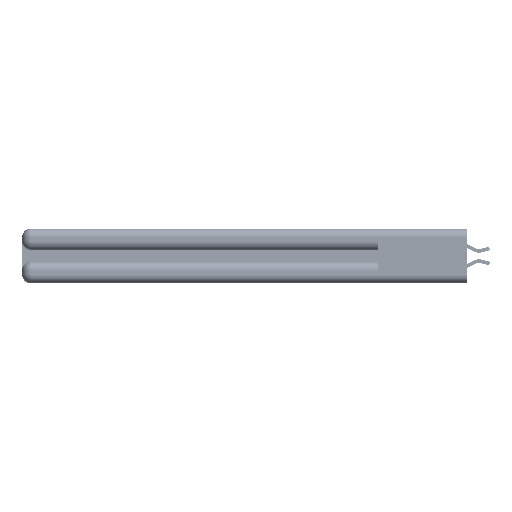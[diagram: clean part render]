
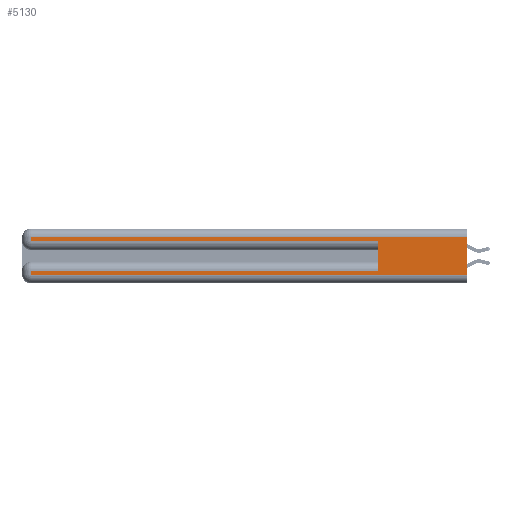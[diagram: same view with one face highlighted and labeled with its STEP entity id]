
A CAD part, left-side view. The second image highlights one B-rep face of the part: STEP entity #5130.
In plain terms, the highlighted planar face has unit normal (-1, 0, 0).
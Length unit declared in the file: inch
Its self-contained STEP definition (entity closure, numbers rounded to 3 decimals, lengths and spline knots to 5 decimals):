
#1641 = VECTOR ( 'NONE', #52643, 39.37008 ) ;
#1784 = VERTEX_POINT ( 'NONE', #21558 ) ;
#3058 = EDGE_CURVE ( 'NONE', #45789, #15807, #40304, .T. ) ;
#3540 = VERTEX_POINT ( 'NONE', #5433 ) ;
#3769 = DIRECTION ( 'NONE',  ( 0., 0., 1. ) ) ;
#5130 = ADVANCED_FACE ( 'NONE', ( #40050 ), #31026, .F. ) ;
#5433 = CARTESIAN_POINT ( 'NONE',  ( 0., 2.94, 0.31 ) ) ;
#5743 = CARTESIAN_POINT ( 'NONE',  ( 0., 2.94, 0.06 ) ) ;
#6105 = CARTESIAN_POINT ( 'NONE',  ( 0., 0.6, 0.285 ) ) ;
#9072 = VECTOR ( 'NONE', #11813, 39.37008 ) ;
#9513 = DIRECTION ( 'NONE',  ( 0., 1., 0. ) ) ;
#10272 = VERTEX_POINT ( 'NONE', #44427 ) ;
#11165 = CARTESIAN_POINT ( 'NONE',  ( 0., 2.94, 0.37 ) ) ;
#11813 = DIRECTION ( 'NONE',  ( 0., -1., 0. ) ) ;
#13017 = CARTESIAN_POINT ( 'NONE',  ( 0., 2.94, 0.085 ) ) ;
#13140 = LINE ( 'NONE', #35290, #1641 ) ;
#13839 = DIRECTION ( 'NONE',  ( 0., 0., -1. ) ) ;
#14484 = EDGE_CURVE ( 'NONE', #3540, #10272, #14761, .T. ) ;
#14699 = DIRECTION ( 'NONE',  ( 0., 1., 0. ) ) ;
#14761 = LINE ( 'NONE', #17998, #22967 ) ;
#15807 = VERTEX_POINT ( 'NONE', #5743 ) ;
#15964 = VECTOR ( 'NONE', #19914, 39.37008 ) ;
#16644 = VECTOR ( 'NONE', #14699, 39.37008 ) ;
#17998 = CARTESIAN_POINT ( 'NONE',  ( 0., 2.94, 0.37 ) ) ;
#18341 = VERTEX_POINT ( 'NONE', #46670 ) ;
#19641 = CARTESIAN_POINT ( 'NONE',  ( 0., 0., 0.37 ) ) ;
#19914 = DIRECTION ( 'NONE',  ( 0., 0., -1. ) ) ;
#20586 = LINE ( 'NONE', #37511, #9072 ) ;
#21558 = CARTESIAN_POINT ( 'NONE',  ( 0., 0., 0.31 ) ) ;
#22157 = LINE ( 'NONE', #19641, #43772 ) ;
#22967 = VECTOR ( 'NONE', #48174, 39.37008 ) ;
#23277 = ORIENTED_EDGE ( 'NONE', *, *, #25528, .T. ) ;
#23896 = ORIENTED_EDGE ( 'NONE', *, *, #39917, .F. ) ;
#23973 = DIRECTION ( 'NONE',  ( 0., 0., -1. ) ) ;
#25344 = CARTESIAN_POINT ( 'NONE',  ( 0., 0.6, 0.145 ) ) ;
#25528 = EDGE_CURVE ( 'NONE', #10272, #27732, #20586, .T. ) ;
#26669 = CARTESIAN_POINT ( 'NONE',  ( 0., 0., 0.06 ) ) ;
#27478 = AXIS2_PLACEMENT_3D ( 'NONE', #35363, #39712, #13839 ) ;
#27732 = VERTEX_POINT ( 'NONE', #6105 ) ;
#28505 = ORIENTED_EDGE ( 'NONE', *, *, #35931, .T. ) ;
#29881 = EDGE_LOOP ( 'NONE', ( #23896, #55010, #33241, #23277, #42672, #37884, #41158, #28505 ) ) ;
#30855 = LINE ( 'NONE', #25344, #36932 ) ;
#30987 = VERTEX_POINT ( 'NONE', #26669 ) ;
#31026 = PLANE ( 'NONE',  #27478 ) ;
#32886 = EDGE_CURVE ( 'NONE', #18341, #27732, #30855, .T. ) ;
#32954 = LINE ( 'NONE', #43890, #54547 ) ;
#33241 = ORIENTED_EDGE ( 'NONE', *, *, #14484, .T. ) ;
#35290 = CARTESIAN_POINT ( 'NONE',  ( 0., 0., 0.06 ) ) ;
#35363 = CARTESIAN_POINT ( 'NONE',  ( 0., 0., 0.37 ) ) ;
#35931 = EDGE_CURVE ( 'NONE', #15807, #30987, #13140, .T. ) ;
#36932 = VECTOR ( 'NONE', #3769, 39.37008 ) ;
#37511 = CARTESIAN_POINT ( 'NONE',  ( 0., 0., 0.285 ) ) ;
#37884 = ORIENTED_EDGE ( 'NONE', *, *, #43105, .T. ) ;
#39712 = DIRECTION ( 'NONE',  ( 1., 0., 0. ) ) ;
#39917 = EDGE_CURVE ( 'NONE', #1784, #30987, #22157, .T. ) ;
#40050 = FACE_OUTER_BOUND ( 'NONE', #29881, .T. ) ;
#40304 = LINE ( 'NONE', #11165, #15964 ) ;
#41158 = ORIENTED_EDGE ( 'NONE', *, *, #3058, .T. ) ;
#42672 = ORIENTED_EDGE ( 'NONE', *, *, #32886, .F. ) ;
#43105 = EDGE_CURVE ( 'NONE', #18341, #45789, #52421, .T. ) ;
#43772 = VECTOR ( 'NONE', #23973, 39.37008 ) ;
#43890 = CARTESIAN_POINT ( 'NONE',  ( 0., 0., 0.31 ) ) ;
#44427 = CARTESIAN_POINT ( 'NONE',  ( 0., 2.94, 0.285 ) ) ;
#44741 = CARTESIAN_POINT ( 'NONE',  ( 0., 0., 0.085 ) ) ;
#45789 = VERTEX_POINT ( 'NONE', #13017 ) ;
#46670 = CARTESIAN_POINT ( 'NONE',  ( 0., 0.6, 0.085 ) ) ;
#48174 = DIRECTION ( 'NONE',  ( 0., 0., -1. ) ) ;
#50151 = EDGE_CURVE ( 'NONE', #1784, #3540, #32954, .T. ) ;
#52421 = LINE ( 'NONE', #44741, #16644 ) ;
#52643 = DIRECTION ( 'NONE',  ( 0., -1., 0. ) ) ;
#54547 = VECTOR ( 'NONE', #9513, 39.37008 ) ;
#55010 = ORIENTED_EDGE ( 'NONE', *, *, #50151, .T. ) ;
